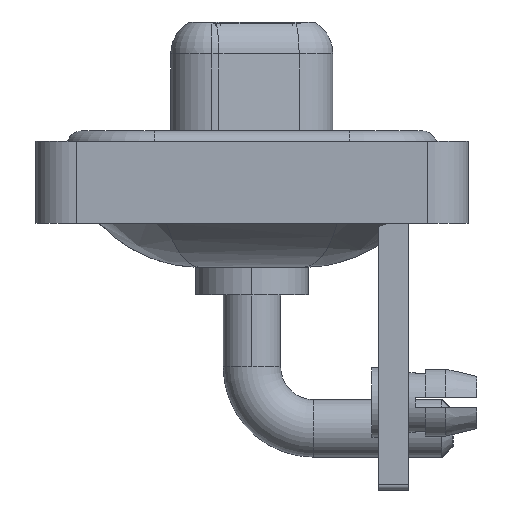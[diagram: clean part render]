
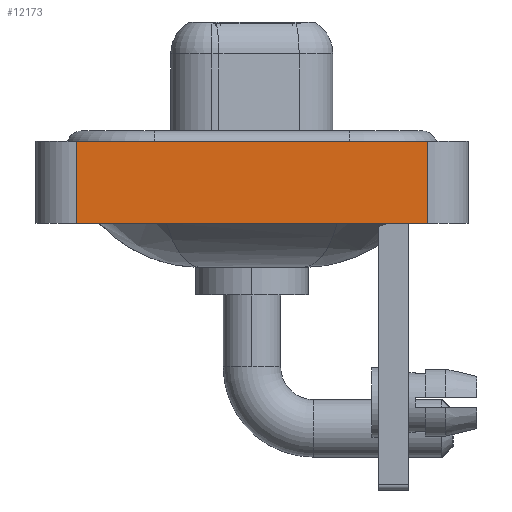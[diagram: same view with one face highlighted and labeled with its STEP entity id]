
A CAD part, left-side view. The second image highlights one B-rep face of the part: STEP entity #12173.
In plain terms, the highlighted planar face has unit normal (-1, 0, 0).
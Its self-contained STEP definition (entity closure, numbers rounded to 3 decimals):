
#1024 = CARTESIAN_POINT ( 'NONE',  ( -7.25, -8.55, -3.6 ) ) ;
#1086 = FACE_OUTER_BOUND ( 'NONE', #2126, .T. ) ;
#1255 = CARTESIAN_POINT ( 'NONE',  ( -7.25, 8.55, -3.6 ) ) ;
#2126 = EDGE_LOOP ( 'NONE', ( #15665, #11488, #9425, #7809 ) ) ;
#2732 = DIRECTION ( 'NONE',  ( 0., -1., 0. ) ) ;
#3410 = CARTESIAN_POINT ( 'NONE',  ( -7.25, -8.55, -3.6 ) ) ;
#5269 = VECTOR ( 'NONE', #14461, 1000. ) ;
#5912 = DIRECTION ( 'NONE',  ( 0., 0., 1. ) ) ;
#6062 = CARTESIAN_POINT ( 'NONE',  ( -7.25, -8.55, -3.6 ) ) ;
#6970 = EDGE_CURVE ( 'NONE', #8265, #13698, #8548, .T. ) ;
#7046 = LINE ( 'NONE', #10273, #14203 ) ;
#7809 = ORIENTED_EDGE ( 'NONE', *, *, #8099, .T. ) ;
#7841 = EDGE_CURVE ( 'NONE', #19138, #13698, #7046, .T. ) ;
#8099 = EDGE_CURVE ( 'NONE', #15776, #8265, #16621, .T. ) ;
#8265 = VERTEX_POINT ( 'NONE', #3410 ) ;
#8548 = LINE ( 'NONE', #1024, #9435 ) ;
#9425 = ORIENTED_EDGE ( 'NONE', *, *, #12818, .F. ) ;
#9435 = VECTOR ( 'NONE', #5912, 1000. ) ;
#10273 = CARTESIAN_POINT ( 'NONE',  ( -7.25, -8.55, 0.4 ) ) ;
#11257 = DIRECTION ( 'NONE',  ( 0., 0., 1. ) ) ;
#11488 = ORIENTED_EDGE ( 'NONE', *, *, #7841, .F. ) ;
#12173 = ADVANCED_FACE ( 'NONE', ( #1086 ), #15568, .T. ) ;
#12619 = VECTOR ( 'NONE', #13399, 1000. ) ;
#12818 = EDGE_CURVE ( 'NONE', #15776, #19138, #13388, .T. ) ;
#12923 = CARTESIAN_POINT ( 'NONE',  ( -7.25, -8.55, -3.6 ) ) ;
#13205 = CARTESIAN_POINT ( 'NONE',  ( -7.25, 8.55, 0.4 ) ) ;
#13357 = CARTESIAN_POINT ( 'NONE',  ( -7.25, 8.55, -3.6 ) ) ;
#13388 = LINE ( 'NONE', #1255, #5269 ) ;
#13399 = DIRECTION ( 'NONE',  ( 0., -1., 0. ) ) ;
#13698 = VERTEX_POINT ( 'NONE', #14889 ) ;
#14203 = VECTOR ( 'NONE', #2732, 1000. ) ;
#14287 = DIRECTION ( 'NONE',  ( -1., 0., 0. ) ) ;
#14461 = DIRECTION ( 'NONE',  ( 0., 0., 1. ) ) ;
#14889 = CARTESIAN_POINT ( 'NONE',  ( -7.25, -8.55, 0.4 ) ) ;
#15568 = PLANE ( 'NONE',  #16802 ) ;
#15665 = ORIENTED_EDGE ( 'NONE', *, *, #6970, .T. ) ;
#15776 = VERTEX_POINT ( 'NONE', #13357 ) ;
#16621 = LINE ( 'NONE', #6062, #12619 ) ;
#16802 = AXIS2_PLACEMENT_3D ( 'NONE', #12923, #14287, #11257 ) ;
#19138 = VERTEX_POINT ( 'NONE', #13205 ) ;
